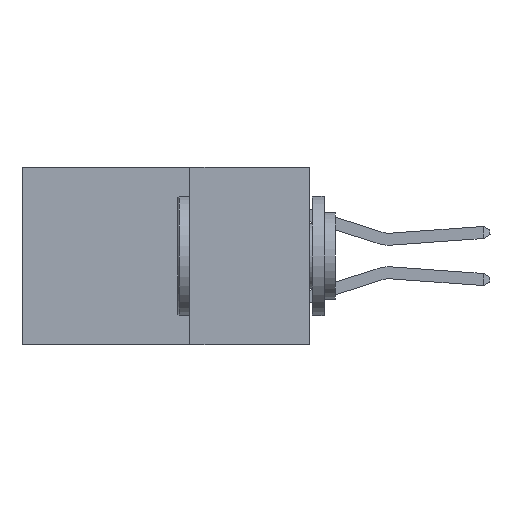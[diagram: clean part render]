
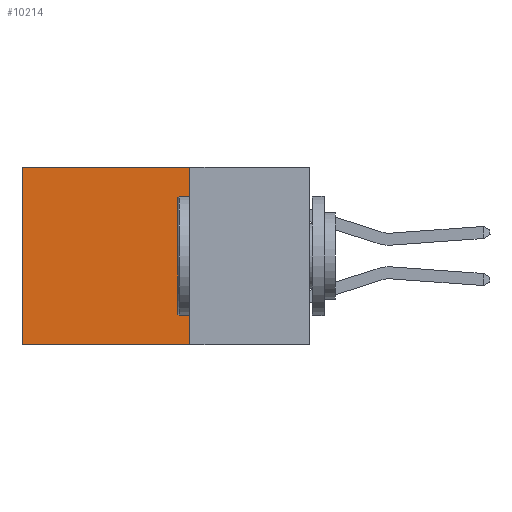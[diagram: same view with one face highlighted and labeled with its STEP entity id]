
A CAD part, left-side view. The second image highlights one B-rep face of the part: STEP entity #10214.
In plain terms, the highlighted planar face has unit normal (-1, 0, 0).
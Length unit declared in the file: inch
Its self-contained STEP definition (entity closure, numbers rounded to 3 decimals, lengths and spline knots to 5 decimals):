
#518 = ORIENTED_EDGE ( 'NONE', *, *, #12649, .T. ) ;
#1904 = ORIENTED_EDGE ( 'NONE', *, *, #10215, .F. ) ;
#2115 = VECTOR ( 'NONE', #13789, 39.37008 ) ;
#3318 = EDGE_CURVE ( 'NONE', #17401, #13826, #14667, .T. ) ;
#3624 = VERTEX_POINT ( 'NONE', #13303 ) ;
#4357 = DIRECTION ( 'NONE',  ( 1., 0., 0. ) ) ;
#4591 = VECTOR ( 'NONE', #13971, 39.37008 ) ;
#6148 = VECTOR ( 'NONE', #23718, 39.37008 ) ;
#6291 = CARTESIAN_POINT ( 'NONE',  ( 0.298, 0.25, 0. ) ) ;
#6721 = CARTESIAN_POINT ( 'NONE',  ( 0.298, 0.6, -0.37 ) ) ;
#7252 = AXIS2_PLACEMENT_3D ( 'NONE', #6291, #4357, #13937 ) ;
#10214 = ADVANCED_FACE ( 'NONE', ( #11256 ), #21216, .F. ) ;
#10215 = EDGE_CURVE ( 'NONE', #3624, #18472, #20634, .T. ) ;
#11071 = EDGE_LOOP ( 'NONE', ( #14914, #17692, #1904, #518 ) ) ;
#11256 = FACE_OUTER_BOUND ( 'NONE', #11071, .T. ) ;
#11704 = CARTESIAN_POINT ( 'NONE',  ( 0.298, 0.25, 0. ) ) ;
#12649 = EDGE_CURVE ( 'NONE', #3624, #17401, #17729, .T. ) ;
#13303 = CARTESIAN_POINT ( 'NONE',  ( 0.298, 0.25, 0. ) ) ;
#13789 = DIRECTION ( 'NONE',  ( 0., 1., 0. ) ) ;
#13826 = VERTEX_POINT ( 'NONE', #6721 ) ;
#13937 = DIRECTION ( 'NONE',  ( 0., 0., -1. ) ) ;
#13971 = DIRECTION ( 'NONE',  ( 0., 1., 0. ) ) ;
#14667 = LINE ( 'NONE', #21590, #6148 ) ;
#14914 = ORIENTED_EDGE ( 'NONE', *, *, #3318, .T. ) ;
#15079 = EDGE_CURVE ( 'NONE', #18472, #13826, #23506, .T. ) ;
#16336 = CARTESIAN_POINT ( 'NONE',  ( 0.298, 0.25, -0.37 ) ) ;
#17401 = VERTEX_POINT ( 'NONE', #24023 ) ;
#17601 = CARTESIAN_POINT ( 'NONE',  ( 0.298, 0.25, -0.37 ) ) ;
#17667 = DIRECTION ( 'NONE',  ( 0., 0., -1. ) ) ;
#17692 = ORIENTED_EDGE ( 'NONE', *, *, #15079, .F. ) ;
#17729 = LINE ( 'NONE', #19593, #4591 ) ;
#18472 = VERTEX_POINT ( 'NONE', #16336 ) ;
#18586 = VECTOR ( 'NONE', #17667, 39.37008 ) ;
#19593 = CARTESIAN_POINT ( 'NONE',  ( 0.298, 0.25, 0. ) ) ;
#20634 = LINE ( 'NONE', #11704, #18586 ) ;
#21216 = PLANE ( 'NONE',  #7252 ) ;
#21590 = CARTESIAN_POINT ( 'NONE',  ( 0.298, 0.6, 0. ) ) ;
#23506 = LINE ( 'NONE', #17601, #2115 ) ;
#23718 = DIRECTION ( 'NONE',  ( 0., 0., -1. ) ) ;
#24023 = CARTESIAN_POINT ( 'NONE',  ( 0.298, 0.6, 0. ) ) ;
